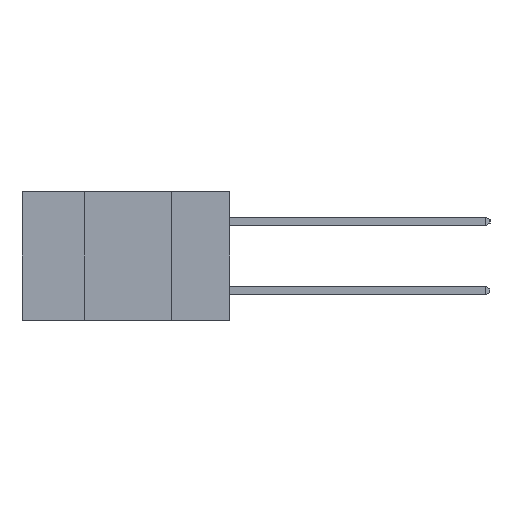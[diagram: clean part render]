
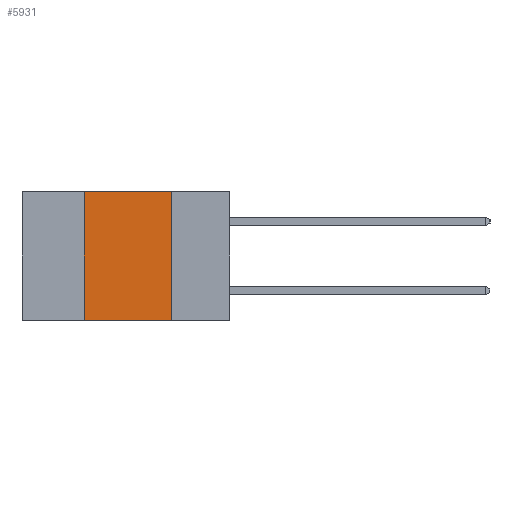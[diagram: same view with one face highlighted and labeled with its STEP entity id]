
A CAD part, left-side view. The second image highlights one B-rep face of the part: STEP entity #5931.
In plain terms, the highlighted planar face has unit normal (-1, 0, 0).
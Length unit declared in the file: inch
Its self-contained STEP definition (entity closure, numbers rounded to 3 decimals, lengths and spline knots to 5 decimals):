
#2110 = LINE ( 'NONE', #23975, #7024 ) ;
#3124 = DIRECTION ( 'NONE',  ( 0., -1., 0. ) ) ;
#3485 = VERTEX_POINT ( 'NONE', #3538 ) ;
#3538 = CARTESIAN_POINT ( 'NONE',  ( 0., 0.42, 0. ) ) ;
#4467 = DIRECTION ( 'NONE',  ( 0., 0., 1. ) ) ;
#4568 = CARTESIAN_POINT ( 'NONE',  ( 0., 0.17, 0. ) ) ;
#4614 = DIRECTION ( 'NONE',  ( 0., 0., -1. ) ) ;
#4678 = DIRECTION ( 'NONE',  ( 1., 0., 0. ) ) ;
#4720 = PLANE ( 'NONE',  #8593 ) ;
#5001 = CARTESIAN_POINT ( 'NONE',  ( 0., 0.6, 0. ) ) ;
#5195 = EDGE_LOOP ( 'NONE', ( #14374, #8997, #18502, #13089 ) ) ;
#5931 = ADVANCED_FACE ( 'NONE', ( #6607 ), #4720, .F. ) ;
#6607 = FACE_OUTER_BOUND ( 'NONE', #5195, .T. ) ;
#7024 = VECTOR ( 'NONE', #7759, 39.37008 ) ;
#7759 = DIRECTION ( 'NONE',  ( 0., -1., 0. ) ) ;
#8593 = AXIS2_PLACEMENT_3D ( 'NONE', #5001, #4678, #4614 ) ;
#8997 = ORIENTED_EDGE ( 'NONE', *, *, #22667, .F. ) ;
#9551 = VERTEX_POINT ( 'NONE', #4568 ) ;
#10716 = CARTESIAN_POINT ( 'NONE',  ( 0., 0.42, -0.37 ) ) ;
#11887 = EDGE_CURVE ( 'NONE', #12097, #14241, #2110, .T. ) ;
#12097 = VERTEX_POINT ( 'NONE', #16293 ) ;
#13089 = ORIENTED_EDGE ( 'NONE', *, *, #11887, .T. ) ;
#13364 = CARTESIAN_POINT ( 'NONE',  ( 0., 0.6, 0. ) ) ;
#13647 = DIRECTION ( 'NONE',  ( 0., 0., -1. ) ) ;
#14241 = VERTEX_POINT ( 'NONE', #14744 ) ;
#14374 = ORIENTED_EDGE ( 'NONE', *, *, #17868, .F. ) ;
#14744 = CARTESIAN_POINT ( 'NONE',  ( 0., 0.17, -0.37 ) ) ;
#15274 = VECTOR ( 'NONE', #4467, 39.37008 ) ;
#15649 = VECTOR ( 'NONE', #13647, 39.37008 ) ;
#16293 = CARTESIAN_POINT ( 'NONE',  ( 0., 0.42, -0.37 ) ) ;
#17868 = EDGE_CURVE ( 'NONE', #9551, #14241, #26528, .T. ) ;
#18498 = LINE ( 'NONE', #13364, #22045 ) ;
#18502 = ORIENTED_EDGE ( 'NONE', *, *, #25890, .F. ) ;
#19882 = CARTESIAN_POINT ( 'NONE',  ( 0., 0.17, -0.37 ) ) ;
#21972 = LINE ( 'NONE', #10716, #15274 ) ;
#22045 = VECTOR ( 'NONE', #3124, 39.37008 ) ;
#22667 = EDGE_CURVE ( 'NONE', #3485, #9551, #18498, .T. ) ;
#23975 = CARTESIAN_POINT ( 'NONE',  ( 0., 0.6, -0.37 ) ) ;
#25890 = EDGE_CURVE ( 'NONE', #12097, #3485, #21972, .T. ) ;
#26528 = LINE ( 'NONE', #19882, #15649 ) ;
